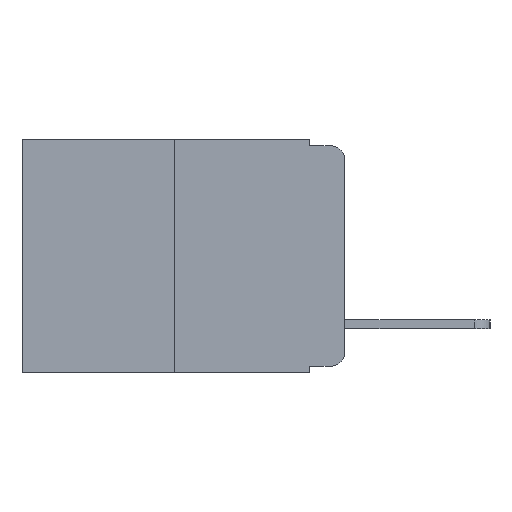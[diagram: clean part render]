
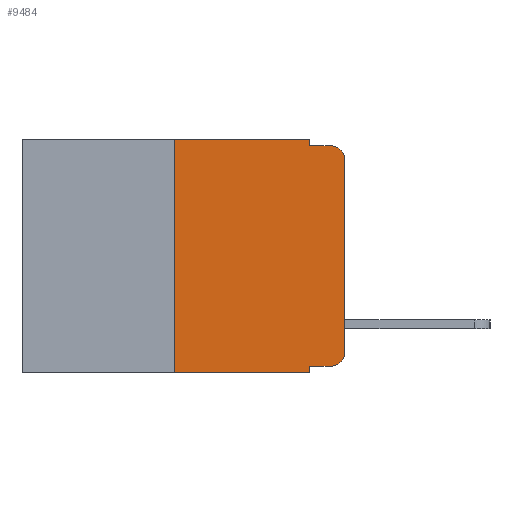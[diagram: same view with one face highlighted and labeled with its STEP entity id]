
A CAD part, left-side view. The second image highlights one B-rep face of the part: STEP entity #9484.
In plain terms, the highlighted planar face has unit normal (-1, 0, 0).
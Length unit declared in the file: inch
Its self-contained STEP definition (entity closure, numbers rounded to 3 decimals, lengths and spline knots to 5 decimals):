
#118 = AXIS2_PLACEMENT_3D ( 'NONE', #24377, #12400, #350 ) ;
#350 = DIRECTION ( 'NONE',  ( 0., 0., -1. ) ) ;
#527 = CARTESIAN_POINT ( 'NONE',  ( 0., 0.02, -0.313 ) ) ;
#686 = ORIENTED_EDGE ( 'NONE', *, *, #9175, .T. ) ;
#931 = DIRECTION ( 'NONE',  ( 0., 0., -1. ) ) ;
#1333 = VERTEX_POINT ( 'NONE', #10640 ) ;
#1442 = LINE ( 'NONE', #10322, #22223 ) ;
#1493 = PLANE ( 'NONE',  #7077 ) ;
#1497 = FACE_OUTER_BOUND ( 'NONE', #4403, .T. ) ;
#1567 = DIRECTION ( 'NONE',  ( 0., 0., -1. ) ) ;
#1615 = LINE ( 'NONE', #10950, #11657 ) ;
#1825 = EDGE_CURVE ( 'NONE', #21842, #4137, #22186, .T. ) ;
#2253 = ORIENTED_EDGE ( 'NONE', *, *, #21737, .F. ) ;
#2327 = EDGE_CURVE ( 'NONE', #20923, #1333, #15589, .T. ) ;
#2554 = DIRECTION ( 'NONE',  ( 0., 0., -1. ) ) ;
#2907 = LINE ( 'NONE', #20324, #8210 ) ;
#3176 = CARTESIAN_POINT ( 'NONE',  ( 0., 0.02, -0.333 ) ) ;
#3177 = ORIENTED_EDGE ( 'NONE', *, *, #1825, .T. ) ;
#3834 = VERTEX_POINT ( 'NONE', #13066 ) ;
#4137 = VERTEX_POINT ( 'NONE', #19958 ) ;
#4181 = VECTOR ( 'NONE', #25108, 39.37008 ) ;
#4403 = EDGE_LOOP ( 'NONE', ( #23903, #3177, #9119, #11028, #17730, #2253, #13625, #25423, #16157, #686 ) ) ;
#5539 = CARTESIAN_POINT ( 'NONE',  ( 0., 0.051, -0.343 ) ) ;
#6087 = VECTOR ( 'NONE', #22998, 39.37008 ) ;
#6301 = EDGE_CURVE ( 'NONE', #1333, #4137, #22236, .T. ) ;
#6536 = LINE ( 'NONE', #10848, #21447 ) ;
#6780 = EDGE_CURVE ( 'NONE', #18007, #20187, #10567, .T. ) ;
#6819 = CARTESIAN_POINT ( 'NONE',  ( 0., 0.051, 0. ) ) ;
#7077 = AXIS2_PLACEMENT_3D ( 'NONE', #11571, #25543, #13666 ) ;
#7115 = CARTESIAN_POINT ( 'NONE',  ( 0., 0.473, 0. ) ) ;
#7993 = EDGE_CURVE ( 'NONE', #15276, #21842, #6536, .T. ) ;
#8142 = DIRECTION ( 'NONE',  ( 0., -1., 0. ) ) ;
#8210 = VECTOR ( 'NONE', #8142, 39.37008 ) ;
#8874 = LINE ( 'NONE', #7115, #4181 ) ;
#9119 = ORIENTED_EDGE ( 'NONE', *, *, #6301, .F. ) ;
#9175 = EDGE_CURVE ( 'NONE', #16371, #15276, #14474, .T. ) ;
#9484 = ADVANCED_FACE ( 'NONE', ( #1497 ), #1493, .F. ) ;
#9783 = CARTESIAN_POINT ( 'NONE',  ( 0., 0.051, 0. ) ) ;
#10322 = CARTESIAN_POINT ( 'NONE',  ( 0., 0.051, -0.333 ) ) ;
#10506 = VERTEX_POINT ( 'NONE', #24736 ) ;
#10567 = LINE ( 'NONE', #6819, #25857 ) ;
#10640 = CARTESIAN_POINT ( 'NONE',  ( 0., 0.051, -0.01 ) ) ;
#10848 = CARTESIAN_POINT ( 'NONE',  ( 0., 0., 0. ) ) ;
#10950 = CARTESIAN_POINT ( 'NONE',  ( 0., 0.25, 0. ) ) ;
#11028 = ORIENTED_EDGE ( 'NONE', *, *, #2327, .F. ) ;
#11427 = EDGE_CURVE ( 'NONE', #10506, #20923, #8874, .T. ) ;
#11571 = CARTESIAN_POINT ( 'NONE',  ( 0., 0.473, 0. ) ) ;
#11657 = VECTOR ( 'NONE', #13022, 39.37008 ) ;
#12400 = DIRECTION ( 'NONE',  ( -1., 0., 0. ) ) ;
#13022 = DIRECTION ( 'NONE',  ( 0., 0., 1. ) ) ;
#13066 = CARTESIAN_POINT ( 'NONE',  ( 0., 0.25, -0.343 ) ) ;
#13375 = CARTESIAN_POINT ( 'NONE',  ( 0., 0., -0.03 ) ) ;
#13625 = ORIENTED_EDGE ( 'NONE', *, *, #20897, .T. ) ;
#13666 = DIRECTION ( 'NONE',  ( 0., 0., -1. ) ) ;
#14474 = CIRCLE ( 'NONE', #22968, 0.02 ) ;
#14663 = DIRECTION ( 'NONE',  ( -1., 0., 0. ) ) ;
#15276 = VERTEX_POINT ( 'NONE', #23346 ) ;
#15589 = LINE ( 'NONE', #9783, #20312 ) ;
#16157 = ORIENTED_EDGE ( 'NONE', *, *, #25287, .T. ) ;
#16371 = VERTEX_POINT ( 'NONE', #3176 ) ;
#17730 = ORIENTED_EDGE ( 'NONE', *, *, #11427, .F. ) ;
#18007 = VERTEX_POINT ( 'NONE', #20175 ) ;
#19958 = CARTESIAN_POINT ( 'NONE',  ( 0., 0.02, -0.01 ) ) ;
#20175 = CARTESIAN_POINT ( 'NONE',  ( 0., 0.051, -0.333 ) ) ;
#20187 = VERTEX_POINT ( 'NONE', #5539 ) ;
#20312 = VECTOR ( 'NONE', #1567, 39.37008 ) ;
#20324 = CARTESIAN_POINT ( 'NONE',  ( 0., 0.473, -0.343 ) ) ;
#20897 = EDGE_CURVE ( 'NONE', #3834, #20187, #2907, .T. ) ;
#20923 = VERTEX_POINT ( 'NONE', #24318 ) ;
#21042 = CARTESIAN_POINT ( 'NONE',  ( 0., 0.051, -0.01 ) ) ;
#21447 = VECTOR ( 'NONE', #22830, 39.37008 ) ;
#21737 = EDGE_CURVE ( 'NONE', #3834, #10506, #1615, .T. ) ;
#21842 = VERTEX_POINT ( 'NONE', #13375 ) ;
#22186 = CIRCLE ( 'NONE', #118, 0.02 ) ;
#22223 = VECTOR ( 'NONE', #24436, 39.37008 ) ;
#22236 = LINE ( 'NONE', #21042, #6087 ) ;
#22830 = DIRECTION ( 'NONE',  ( 0., 0., 1. ) ) ;
#22968 = AXIS2_PLACEMENT_3D ( 'NONE', #527, #14663, #2554 ) ;
#22998 = DIRECTION ( 'NONE',  ( 0., -1., 0. ) ) ;
#23346 = CARTESIAN_POINT ( 'NONE',  ( 0., 0., -0.313 ) ) ;
#23903 = ORIENTED_EDGE ( 'NONE', *, *, #7993, .T. ) ;
#24318 = CARTESIAN_POINT ( 'NONE',  ( 0., 0.051, 0. ) ) ;
#24377 = CARTESIAN_POINT ( 'NONE',  ( 0., 0.02, -0.03 ) ) ;
#24436 = DIRECTION ( 'NONE',  ( 0., -1., 0. ) ) ;
#24736 = CARTESIAN_POINT ( 'NONE',  ( 0., 0.25, 0. ) ) ;
#25108 = DIRECTION ( 'NONE',  ( 0., -1., 0. ) ) ;
#25287 = EDGE_CURVE ( 'NONE', #18007, #16371, #1442, .T. ) ;
#25423 = ORIENTED_EDGE ( 'NONE', *, *, #6780, .F. ) ;
#25543 = DIRECTION ( 'NONE',  ( 1., 0., 0. ) ) ;
#25857 = VECTOR ( 'NONE', #931, 39.37008 ) ;
